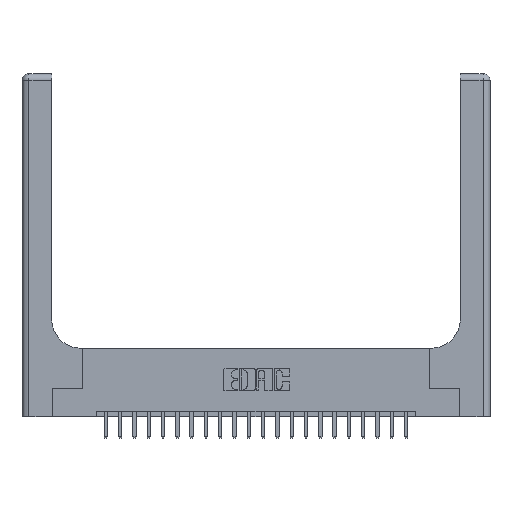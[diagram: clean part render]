
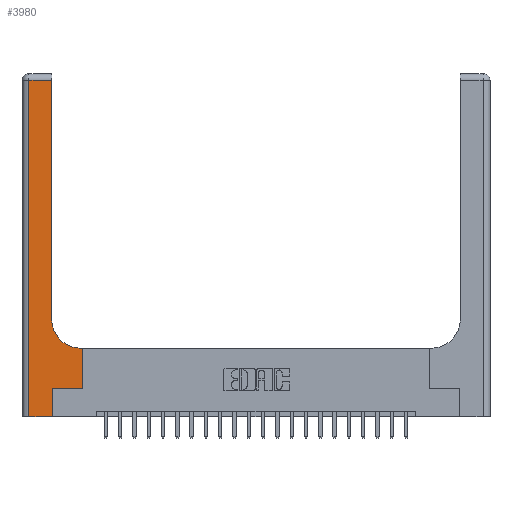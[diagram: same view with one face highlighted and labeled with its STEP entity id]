
A CAD part, top view. The second image highlights one B-rep face of the part: STEP entity #3980.
In plain terms, the highlighted planar face has unit normal (0, 0, 1).
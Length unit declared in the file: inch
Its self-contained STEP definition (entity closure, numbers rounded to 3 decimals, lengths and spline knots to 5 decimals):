
#24 = EDGE_CURVE ( 'NONE', #20826, #17548, #11481, .T. ) ;
#186 = ORIENTED_EDGE ( 'NONE', *, *, #16475, .T. ) ;
#934 = AXIS2_PLACEMENT_3D ( 'NONE', #17287, #17053, #4933 ) ;
#1013 = LINE ( 'NONE', #13255, #11019 ) ;
#1209 = DIRECTION ( 'NONE',  ( -1., 0., 0. ) ) ;
#1312 = VECTOR ( 'NONE', #10157, 39.37008 ) ;
#1431 = CARTESIAN_POINT ( 'NONE',  ( 0.528, 0.6, 0.37 ) ) ;
#1643 = CARTESIAN_POINT ( 'NONE',  ( 0., 0., 0.37 ) ) ;
#1682 = CARTESIAN_POINT ( 'NONE',  ( 0.06, 0., 0.37 ) ) ;
#1811 = EDGE_CURVE ( 'NONE', #9065, #9271, #15301, .T. ) ;
#1983 = ORIENTED_EDGE ( 'NONE', *, *, #22741, .T. ) ;
#2228 = PLANE ( 'NONE',  #12919 ) ;
#2596 = ORIENTED_EDGE ( 'NONE', *, *, #24, .T. ) ;
#2669 = DIRECTION ( 'NONE',  ( 0., 1., 0. ) ) ;
#3015 = LINE ( 'NONE', #22273, #13803 ) ;
#3642 = EDGE_LOOP ( 'NONE', ( #5006, #15346, #15205, #4490, #186, #1983, #5115, #2596, #17175 ) ) ;
#3908 = LINE ( 'NONE', #5869, #7150 ) ;
#3980 = ADVANCED_FACE ( 'NONE', ( #7892 ), #2228, .F. ) ;
#4127 = VECTOR ( 'NONE', #9157, 39.37008 ) ;
#4361 = DIRECTION ( 'NONE',  ( -1., 0., 0. ) ) ;
#4428 = CARTESIAN_POINT ( 'NONE',  ( 0.26, 0.85, 0.37 ) ) ;
#4490 = ORIENTED_EDGE ( 'NONE', *, *, #1811, .T. ) ;
#4933 = DIRECTION ( 'NONE',  ( 1., 0., 0. ) ) ;
#4978 = CARTESIAN_POINT ( 'NONE',  ( 0.265, 0.25, 0.37 ) ) ;
#4992 = VECTOR ( 'NONE', #22328, 39.37008 ) ;
#5006 = ORIENTED_EDGE ( 'NONE', *, *, #8404, .T. ) ;
#5115 = ORIENTED_EDGE ( 'NONE', *, *, #11762, .T. ) ;
#5528 = VERTEX_POINT ( 'NONE', #11429 ) ;
#5869 = CARTESIAN_POINT ( 'NONE',  ( 0., 2.94, 0.37 ) ) ;
#6056 = VERTEX_POINT ( 'NONE', #13258 ) ;
#7150 = VECTOR ( 'NONE', #4361, 39.37008 ) ;
#7322 = CARTESIAN_POINT ( 'NONE',  ( 0.265, 0., 0.37 ) ) ;
#7463 = EDGE_CURVE ( 'NONE', #5528, #9065, #1013, .T. ) ;
#7892 = FACE_OUTER_BOUND ( 'NONE', #3642, .T. ) ;
#8404 = EDGE_CURVE ( 'NONE', #13616, #6056, #3015, .T. ) ;
#9065 = VERTEX_POINT ( 'NONE', #1682 ) ;
#9157 = DIRECTION ( 'NONE',  ( 0., 1., 0. ) ) ;
#9271 = VERTEX_POINT ( 'NONE', #13543 ) ;
#10157 = DIRECTION ( 'NONE',  ( 1., 0., 0. ) ) ;
#10608 = CARTESIAN_POINT ( 'NONE',  ( 0.528, 0.25, 0.37 ) ) ;
#10915 = DIRECTION ( 'NONE',  ( 0., 1., 0. ) ) ;
#11019 = VECTOR ( 'NONE', #18900, 39.37008 ) ;
#11429 = CARTESIAN_POINT ( 'NONE',  ( 0.06, 2.94, 0.37 ) ) ;
#11481 = LINE ( 'NONE', #18749, #14883 ) ;
#11762 = EDGE_CURVE ( 'NONE', #17264, #20826, #21296, .T. ) ;
#12554 = CARTESIAN_POINT ( 'NONE',  ( 0.265, 0.25, 0.37 ) ) ;
#12628 = DIRECTION ( 'NONE',  ( -1., 0., 0. ) ) ;
#12919 = AXIS2_PLACEMENT_3D ( 'NONE', #20111, #14914, #12628 ) ;
#13255 = CARTESIAN_POINT ( 'NONE',  ( 0.06, 3., 0.37 ) ) ;
#13258 = CARTESIAN_POINT ( 'NONE',  ( 0.26, 2.94, 0.37 ) ) ;
#13543 = CARTESIAN_POINT ( 'NONE',  ( 0.265, 0., 0.37 ) ) ;
#13616 = VERTEX_POINT ( 'NONE', #4428 ) ;
#13741 = LINE ( 'NONE', #4978, #1312 ) ;
#13803 = VECTOR ( 'NONE', #2669, 39.37008 ) ;
#14324 = VERTEX_POINT ( 'NONE', #12554 ) ;
#14883 = VECTOR ( 'NONE', #1209, 39.37008 ) ;
#14914 = DIRECTION ( 'NONE',  ( 0., 0., -1. ) ) ;
#15205 = ORIENTED_EDGE ( 'NONE', *, *, #7463, .T. ) ;
#15301 = LINE ( 'NONE', #1643, #4992 ) ;
#15346 = ORIENTED_EDGE ( 'NONE', *, *, #18736, .T. ) ;
#16305 = LINE ( 'NONE', #7322, #4127 ) ;
#16475 = EDGE_CURVE ( 'NONE', #9271, #14324, #16305, .T. ) ;
#17053 = DIRECTION ( 'NONE',  ( 0., 0., -1. ) ) ;
#17175 = ORIENTED_EDGE ( 'NONE', *, *, #20349, .T. ) ;
#17264 = VERTEX_POINT ( 'NONE', #10608 ) ;
#17287 = CARTESIAN_POINT ( 'NONE',  ( 0.51, 0.85, 0.37 ) ) ;
#17548 = VERTEX_POINT ( 'NONE', #19091 ) ;
#18736 = EDGE_CURVE ( 'NONE', #6056, #5528, #3908, .T. ) ;
#18749 = CARTESIAN_POINT ( 'NONE',  ( 0.26, 0.6, 0.37 ) ) ;
#18900 = DIRECTION ( 'NONE',  ( 0., -1., 0. ) ) ;
#19091 = CARTESIAN_POINT ( 'NONE',  ( 0.51, 0.6, 0.37 ) ) ;
#19459 = CARTESIAN_POINT ( 'NONE',  ( 0.528, 0.25, 0.37 ) ) ;
#20111 = CARTESIAN_POINT ( 'NONE',  ( 0., 3., 0.37 ) ) ;
#20349 = EDGE_CURVE ( 'NONE', #17548, #13616, #22659, .T. ) ;
#20826 = VERTEX_POINT ( 'NONE', #1431 ) ;
#20967 = VECTOR ( 'NONE', #10915, 39.37008 ) ;
#21296 = LINE ( 'NONE', #19459, #20967 ) ;
#22273 = CARTESIAN_POINT ( 'NONE',  ( 0.26, 3., 0.37 ) ) ;
#22328 = DIRECTION ( 'NONE',  ( 1., 0., 0. ) ) ;
#22659 = CIRCLE ( 'NONE', #934, 0.25 ) ;
#22741 = EDGE_CURVE ( 'NONE', #14324, #17264, #13741, .T. ) ;
